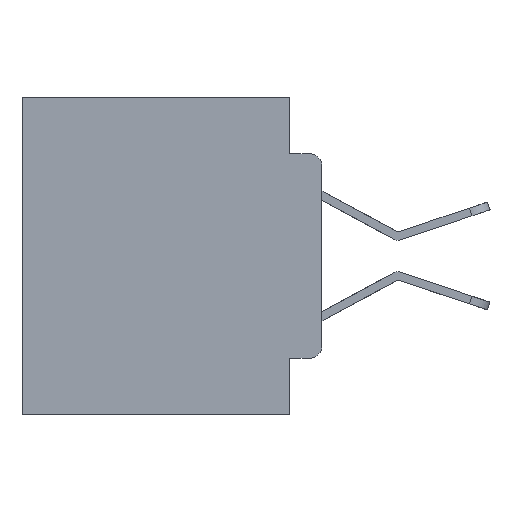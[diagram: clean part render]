
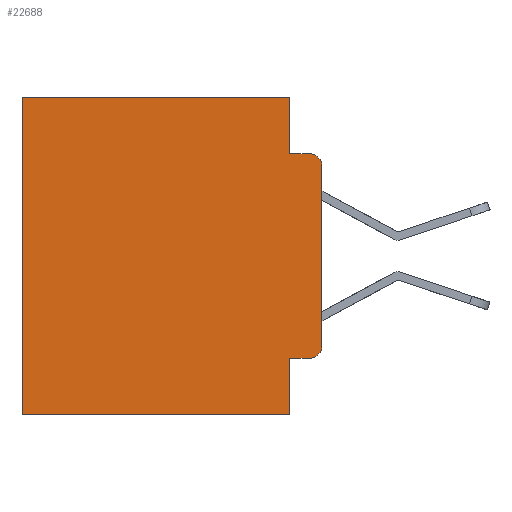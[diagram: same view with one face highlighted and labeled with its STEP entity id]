
A CAD part, left-side view. The second image highlights one B-rep face of the part: STEP entity #22688.
In plain terms, the highlighted planar face has unit normal (-1, 0, 0).
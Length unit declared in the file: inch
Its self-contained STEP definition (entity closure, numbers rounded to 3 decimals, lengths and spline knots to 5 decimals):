
#136 = EDGE_CURVE ( 'NONE', #379, #3839, #25685, .T. ) ;
#357 = DIRECTION ( 'NONE',  ( 0., -1., 0. ) ) ;
#379 = VERTEX_POINT ( 'NONE', #22603 ) ;
#651 = CARTESIAN_POINT ( 'NONE',  ( 0.298, 0.051, -0.0885 ) ) ;
#995 = CARTESIAN_POINT ( 'NONE',  ( 0.298, 0., -0.3915 ) ) ;
#1071 = ORIENTED_EDGE ( 'NONE', *, *, #19792, .F. ) ;
#1217 = VECTOR ( 'NONE', #13907, 39.37008 ) ;
#1360 = EDGE_CURVE ( 'NONE', #9853, #8321, #6490, .T. ) ;
#2004 = VERTEX_POINT ( 'NONE', #3553 ) ;
#2076 = VERTEX_POINT ( 'NONE', #13825 ) ;
#2114 = CARTESIAN_POINT ( 'NONE',  ( 0.298, 0.473, 0. ) ) ;
#2891 = DIRECTION ( 'NONE',  ( 0., 0., -1. ) ) ;
#3187 = DIRECTION ( 'NONE',  ( -1., 0., 0. ) ) ;
#3324 = EDGE_CURVE ( 'NONE', #8321, #14279, #15912, .T. ) ;
#3553 = CARTESIAN_POINT ( 'NONE',  ( 0.298, 0.473, -0.5 ) ) ;
#3672 = ORIENTED_EDGE ( 'NONE', *, *, #136, .F. ) ;
#3829 = CARTESIAN_POINT ( 'NONE',  ( 0.298, 0., 0. ) ) ;
#3839 = VERTEX_POINT ( 'NONE', #651 ) ;
#4310 = EDGE_CURVE ( 'NONE', #3839, #7642, #14592, .T. ) ;
#4467 = DIRECTION ( 'NONE',  ( 0., 0., -1. ) ) ;
#4970 = CARTESIAN_POINT ( 'NONE',  ( 0.298, 0.051, 0. ) ) ;
#5057 = CARTESIAN_POINT ( 'NONE',  ( 0.298, 0., 0. ) ) ;
#5154 = DIRECTION ( 'NONE',  ( 0., 0., -1. ) ) ;
#5195 = VECTOR ( 'NONE', #11205, 39.37008 ) ;
#5327 = CARTESIAN_POINT ( 'NONE',  ( 0.298, 0.051, -0.0885 ) ) ;
#5948 = DIRECTION ( 'NONE',  ( 0., 0., -1. ) ) ;
#6457 = EDGE_CURVE ( 'NONE', #379, #19177, #12263, .T. ) ;
#6458 = DIRECTION ( 'NONE',  ( 0., -1., 0. ) ) ;
#6490 = LINE ( 'NONE', #10104, #16760 ) ;
#6931 = ORIENTED_EDGE ( 'NONE', *, *, #17018, .F. ) ;
#7642 = VERTEX_POINT ( 'NONE', #26054 ) ;
#7757 = LINE ( 'NONE', #3829, #24621 ) ;
#8321 = VERTEX_POINT ( 'NONE', #20030 ) ;
#8560 = DIRECTION ( 'NONE',  ( 0., 0., -1. ) ) ;
#8571 = ORIENTED_EDGE ( 'NONE', *, *, #6457, .T. ) ;
#9131 = CARTESIAN_POINT ( 'NONE',  ( 0.298, 0.473, 0. ) ) ;
#9534 = VECTOR ( 'NONE', #2891, 39.37008 ) ;
#9853 = VERTEX_POINT ( 'NONE', #20918 ) ;
#10104 = CARTESIAN_POINT ( 'NONE',  ( 0.298, 0.051, -0.4115 ) ) ;
#10307 = EDGE_LOOP ( 'NONE', ( #6931, #21910, #10538, #3672, #8571, #12754, #22880, #1071, #20646, #24751 ) ) ;
#10347 = AXIS2_PLACEMENT_3D ( 'NONE', #15541, #3187, #17558 ) ;
#10430 = LINE ( 'NONE', #22430, #25933 ) ;
#10538 = ORIENTED_EDGE ( 'NONE', *, *, #4310, .F. ) ;
#10632 = EDGE_CURVE ( 'NONE', #2076, #2004, #10430, .T. ) ;
#10790 = EDGE_CURVE ( 'NONE', #19177, #2004, #21482, .T. ) ;
#11205 = DIRECTION ( 'NONE',  ( 0., 0., -1. ) ) ;
#12263 = LINE ( 'NONE', #19928, #1217 ) ;
#12754 = ORIENTED_EDGE ( 'NONE', *, *, #10790, .T. ) ;
#12926 = CARTESIAN_POINT ( 'NONE',  ( 0.298, 0., -0.1085 ) ) ;
#13825 = CARTESIAN_POINT ( 'NONE',  ( 0.298, 0.051, -0.5 ) ) ;
#13907 = DIRECTION ( 'NONE',  ( 0., 1., 0. ) ) ;
#13944 = DIRECTION ( 'NONE',  ( -1., 0., 0. ) ) ;
#14279 = VERTEX_POINT ( 'NONE', #995 ) ;
#14323 = AXIS2_PLACEMENT_3D ( 'NONE', #5057, #17425, #5154 ) ;
#14592 = LINE ( 'NONE', #5327, #19353 ) ;
#14747 = CARTESIAN_POINT ( 'NONE',  ( 0.298, 0.051, 0. ) ) ;
#14929 = CARTESIAN_POINT ( 'NONE',  ( 0.298, 0.02, -0.3915 ) ) ;
#15427 = PLANE ( 'NONE',  #14323 ) ;
#15541 = CARTESIAN_POINT ( 'NONE',  ( 0.298, 0.02, -0.1085 ) ) ;
#15912 = CIRCLE ( 'NONE', #24603, 0.02 ) ;
#16287 = LINE ( 'NONE', #14747, #21025 ) ;
#16349 = DIRECTION ( 'NONE',  ( 0., 1., 0. ) ) ;
#16651 = VERTEX_POINT ( 'NONE', #12926 ) ;
#16760 = VECTOR ( 'NONE', #6458, 39.37008 ) ;
#17018 = EDGE_CURVE ( 'NONE', #16651, #14279, #7757, .T. ) ;
#17425 = DIRECTION ( 'NONE',  ( 1., 0., 0. ) ) ;
#17558 = DIRECTION ( 'NONE',  ( 0., 0., -1. ) ) ;
#19177 = VERTEX_POINT ( 'NONE', #2114 ) ;
#19353 = VECTOR ( 'NONE', #357, 39.37008 ) ;
#19792 = EDGE_CURVE ( 'NONE', #9853, #2076, #16287, .T. ) ;
#19928 = CARTESIAN_POINT ( 'NONE',  ( 0.298, 0., 0. ) ) ;
#20012 = EDGE_CURVE ( 'NONE', #16651, #7642, #21325, .T. ) ;
#20030 = CARTESIAN_POINT ( 'NONE',  ( 0.298, 0.02, -0.4115 ) ) ;
#20646 = ORIENTED_EDGE ( 'NONE', *, *, #1360, .T. ) ;
#20918 = CARTESIAN_POINT ( 'NONE',  ( 0.298, 0.051, -0.4115 ) ) ;
#21025 = VECTOR ( 'NONE', #4467, 39.37008 ) ;
#21325 = CIRCLE ( 'NONE', #10347, 0.02 ) ;
#21482 = LINE ( 'NONE', #9131, #5195 ) ;
#21910 = ORIENTED_EDGE ( 'NONE', *, *, #20012, .T. ) ;
#22430 = CARTESIAN_POINT ( 'NONE',  ( 0.298, 0., -0.5 ) ) ;
#22603 = CARTESIAN_POINT ( 'NONE',  ( 0.298, 0.051, 0. ) ) ;
#22688 = ADVANCED_FACE ( 'NONE', ( #25158 ), #15427, .F. ) ;
#22880 = ORIENTED_EDGE ( 'NONE', *, *, #10632, .F. ) ;
#24603 = AXIS2_PLACEMENT_3D ( 'NONE', #14929, #13944, #8560 ) ;
#24621 = VECTOR ( 'NONE', #5948, 39.37008 ) ;
#24751 = ORIENTED_EDGE ( 'NONE', *, *, #3324, .T. ) ;
#25158 = FACE_OUTER_BOUND ( 'NONE', #10307, .T. ) ;
#25685 = LINE ( 'NONE', #4970, #9534 ) ;
#25933 = VECTOR ( 'NONE', #16349, 39.37008 ) ;
#26054 = CARTESIAN_POINT ( 'NONE',  ( 0.298, 0.02, -0.0885 ) ) ;
